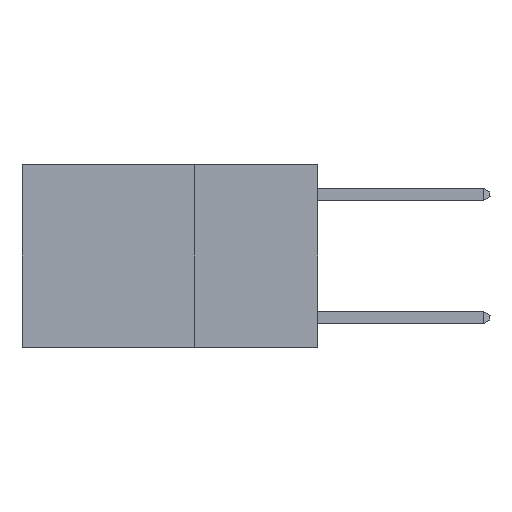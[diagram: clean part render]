
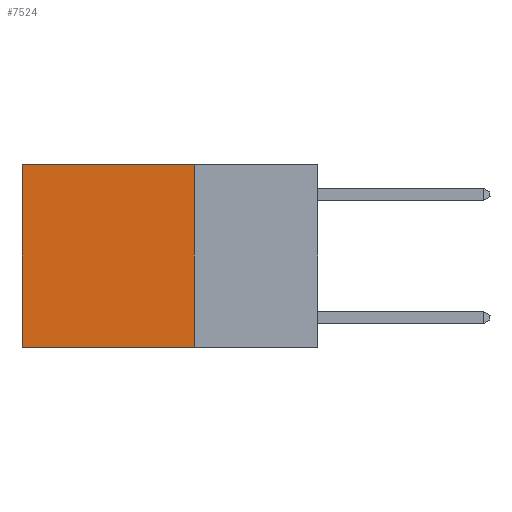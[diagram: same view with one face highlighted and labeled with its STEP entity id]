
A CAD part, left-side view. The second image highlights one B-rep face of the part: STEP entity #7524.
In plain terms, the highlighted planar face has unit normal (-1, 0, 0).
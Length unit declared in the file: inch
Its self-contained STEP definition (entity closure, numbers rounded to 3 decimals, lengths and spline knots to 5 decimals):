
#276 = DIRECTION ( 'NONE',  ( 1., 0., 0. ) ) ;
#2972 = LINE ( 'NONE', #6498, #5905 ) ;
#3103 = VERTEX_POINT ( 'NONE', #11946 ) ;
#3126 = VERTEX_POINT ( 'NONE', #10367 ) ;
#3371 = EDGE_CURVE ( 'NONE', #3126, #13554, #8006, .T. ) ;
#3688 = VERTEX_POINT ( 'NONE', #5186 ) ;
#3749 = DIRECTION ( 'NONE',  ( 0., 1., 0. ) ) ;
#3903 = AXIS2_PLACEMENT_3D ( 'NONE', #9742, #276, #9621 ) ;
#4151 = EDGE_CURVE ( 'NONE', #3103, #13554, #10266, .T. ) ;
#4264 = ORIENTED_EDGE ( 'NONE', *, *, #14232, .T. ) ;
#5154 = EDGE_LOOP ( 'NONE', ( #5785, #13349, #6656, #4264 ) ) ;
#5186 = CARTESIAN_POINT ( 'NONE',  ( 0.2625, 0.25, 0. ) ) ;
#5785 = ORIENTED_EDGE ( 'NONE', *, *, #3371, .T. ) ;
#5905 = VECTOR ( 'NONE', #11827, 39.37008 ) ;
#6498 = CARTESIAN_POINT ( 'NONE',  ( 0.2625, 0.25, 0. ) ) ;
#6656 = ORIENTED_EDGE ( 'NONE', *, *, #10546, .F. ) ;
#7156 = CARTESIAN_POINT ( 'NONE',  ( 0.2625, 0.25, 0. ) ) ;
#7524 = ADVANCED_FACE ( 'NONE', ( #15186 ), #8276, .F. ) ;
#7885 = LINE ( 'NONE', #7156, #14565 ) ;
#8006 = LINE ( 'NONE', #13637, #10518 ) ;
#8276 = PLANE ( 'NONE',  #3903 ) ;
#9621 = DIRECTION ( 'NONE',  ( 0., 0., -1. ) ) ;
#9732 = DIRECTION ( 'NONE',  ( 0., 1., 0. ) ) ;
#9742 = CARTESIAN_POINT ( 'NONE',  ( 0.2625, 0.25, 0. ) ) ;
#10007 = DIRECTION ( 'NONE',  ( 0., 0., -1. ) ) ;
#10266 = LINE ( 'NONE', #15941, #10679 ) ;
#10367 = CARTESIAN_POINT ( 'NONE',  ( 0.2625, 0.6, 0. ) ) ;
#10518 = VECTOR ( 'NONE', #10007, 39.37008 ) ;
#10546 = EDGE_CURVE ( 'NONE', #3688, #3103, #2972, .T. ) ;
#10679 = VECTOR ( 'NONE', #3749, 39.37008 ) ;
#10877 = CARTESIAN_POINT ( 'NONE',  ( 0.2625, 0.6, -0.37 ) ) ;
#11827 = DIRECTION ( 'NONE',  ( 0., 0., -1. ) ) ;
#11946 = CARTESIAN_POINT ( 'NONE',  ( 0.2625, 0.25, -0.37 ) ) ;
#13349 = ORIENTED_EDGE ( 'NONE', *, *, #4151, .F. ) ;
#13554 = VERTEX_POINT ( 'NONE', #10877 ) ;
#13637 = CARTESIAN_POINT ( 'NONE',  ( 0.2625, 0.6, 0. ) ) ;
#14232 = EDGE_CURVE ( 'NONE', #3688, #3126, #7885, .T. ) ;
#14565 = VECTOR ( 'NONE', #9732, 39.37008 ) ;
#15186 = FACE_OUTER_BOUND ( 'NONE', #5154, .T. ) ;
#15941 = CARTESIAN_POINT ( 'NONE',  ( 0.2625, 0.25, -0.37 ) ) ;
